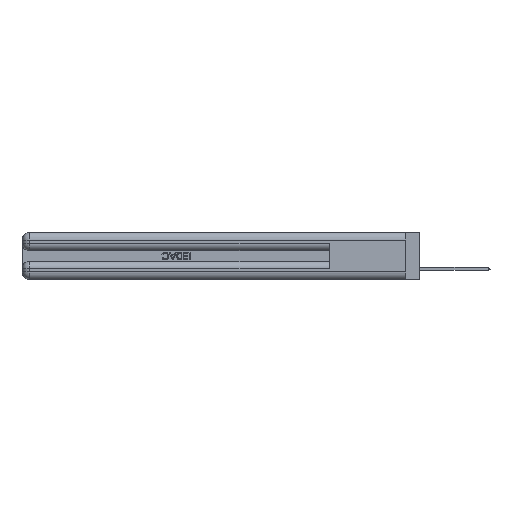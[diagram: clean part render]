
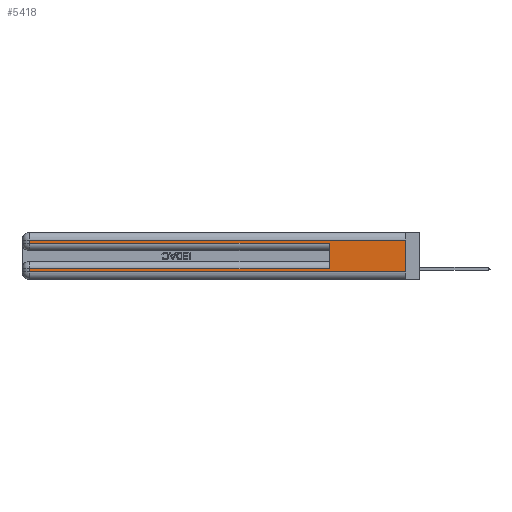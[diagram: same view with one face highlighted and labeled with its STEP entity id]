
A CAD part, left-side view. The second image highlights one B-rep face of the part: STEP entity #5418.
In plain terms, the highlighted planar face has unit normal (-1, 0, 0).
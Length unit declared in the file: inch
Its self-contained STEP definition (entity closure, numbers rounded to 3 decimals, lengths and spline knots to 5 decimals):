
#578 = CARTESIAN_POINT ( 'NONE',  ( 0., 0., 0.31 ) ) ;
#2004 = CARTESIAN_POINT ( 'NONE',  ( 0., 0., 0.06 ) ) ;
#3283 = ORIENTED_EDGE ( 'NONE', *, *, #33619, .F. ) ;
#3835 = CARTESIAN_POINT ( 'NONE',  ( 0., 2.94, 0.085 ) ) ;
#4847 = CARTESIAN_POINT ( 'NONE',  ( 0., 0.6, 0.145 ) ) ;
#4891 = FACE_OUTER_BOUND ( 'NONE', #30828, .T. ) ;
#5418 = ADVANCED_FACE ( 'NONE', ( #4891 ), #45806, .F. ) ;
#5597 = LINE ( 'NONE', #6065, #46303 ) ;
#5659 = ORIENTED_EDGE ( 'NONE', *, *, #11687, .T. ) ;
#6065 = CARTESIAN_POINT ( 'NONE',  ( 0., 0., 0.06 ) ) ;
#8136 = CARTESIAN_POINT ( 'NONE',  ( 0., 0.6, 0.285 ) ) ;
#8319 = DIRECTION ( 'NONE',  ( 0., -1., 0. ) ) ;
#9728 = DIRECTION ( 'NONE',  ( 0., -1., 0. ) ) ;
#9933 = ORIENTED_EDGE ( 'NONE', *, *, #39784, .T. ) ;
#10001 = EDGE_CURVE ( 'NONE', #17465, #18333, #43535, .T. ) ;
#10147 = DIRECTION ( 'NONE',  ( 0., 0., -1. ) ) ;
#11687 = EDGE_CURVE ( 'NONE', #16791, #30083, #5597, .T. ) ;
#12102 = EDGE_CURVE ( 'NONE', #19989, #16791, #15691, .T. ) ;
#12674 = ORIENTED_EDGE ( 'NONE', *, *, #14709, .T. ) ;
#13587 = CARTESIAN_POINT ( 'NONE',  ( 0., 0., 0.37 ) ) ;
#14413 = CARTESIAN_POINT ( 'NONE',  ( 0., 2.94, 0.31 ) ) ;
#14709 = EDGE_CURVE ( 'NONE', #17465, #19989, #40581, .T. ) ;
#15691 = LINE ( 'NONE', #34721, #22446 ) ;
#15802 = EDGE_CURVE ( 'NONE', #34759, #30915, #16139, .T. ) ;
#16139 = LINE ( 'NONE', #44559, #42785 ) ;
#16165 = DIRECTION ( 'NONE',  ( 0., 1., 0. ) ) ;
#16599 = ORIENTED_EDGE ( 'NONE', *, *, #10001, .F. ) ;
#16791 = VERTEX_POINT ( 'NONE', #44982 ) ;
#17465 = VERTEX_POINT ( 'NONE', #32274 ) ;
#18333 = VERTEX_POINT ( 'NONE', #8136 ) ;
#18549 = ORIENTED_EDGE ( 'NONE', *, *, #39634, .T. ) ;
#19989 = VERTEX_POINT ( 'NONE', #3835 ) ;
#21308 = VECTOR ( 'NONE', #35297, 39.37008 ) ;
#21739 = DIRECTION ( 'NONE',  ( 0., 1., 0. ) ) ;
#22446 = VECTOR ( 'NONE', #45543, 39.37008 ) ;
#22933 = DIRECTION ( 'NONE',  ( 0., 0., -1. ) ) ;
#26005 = CARTESIAN_POINT ( 'NONE',  ( 0., 0., 0.285 ) ) ;
#26171 = DIRECTION ( 'NONE',  ( 0., 0., 1. ) ) ;
#26595 = VECTOR ( 'NONE', #26171, 39.37008 ) ;
#27523 = DIRECTION ( 'NONE',  ( 1., 0., 0. ) ) ;
#28692 = LINE ( 'NONE', #13587, #21308 ) ;
#29706 = CARTESIAN_POINT ( 'NONE',  ( 0., 2.94, 0.285 ) ) ;
#30083 = VERTEX_POINT ( 'NONE', #2004 ) ;
#30324 = LINE ( 'NONE', #31939, #45590 ) ;
#30828 = EDGE_LOOP ( 'NONE', ( #3283, #9933, #41014, #18549, #16599, #12674, #33425, #5659 ) ) ;
#30915 = VERTEX_POINT ( 'NONE', #29706 ) ;
#31939 = CARTESIAN_POINT ( 'NONE',  ( 0., 0., 0.31 ) ) ;
#32274 = CARTESIAN_POINT ( 'NONE',  ( 0., 0.6, 0.085 ) ) ;
#33425 = ORIENTED_EDGE ( 'NONE', *, *, #12102, .T. ) ;
#33619 = EDGE_CURVE ( 'NONE', #46067, #30083, #28692, .T. ) ;
#33727 = LINE ( 'NONE', #26005, #44964 ) ;
#34721 = CARTESIAN_POINT ( 'NONE',  ( 0., 2.94, 0.37 ) ) ;
#34759 = VERTEX_POINT ( 'NONE', #14413 ) ;
#35297 = DIRECTION ( 'NONE',  ( 0., 0., -1. ) ) ;
#37685 = CARTESIAN_POINT ( 'NONE',  ( 0., 0., 0.085 ) ) ;
#38572 = CARTESIAN_POINT ( 'NONE',  ( 0., 0., 0.37 ) ) ;
#39634 = EDGE_CURVE ( 'NONE', #30915, #18333, #33727, .T. ) ;
#39784 = EDGE_CURVE ( 'NONE', #46067, #34759, #30324, .T. ) ;
#40581 = LINE ( 'NONE', #37685, #42331 ) ;
#41014 = ORIENTED_EDGE ( 'NONE', *, *, #15802, .T. ) ;
#42331 = VECTOR ( 'NONE', #16165, 39.37008 ) ;
#42785 = VECTOR ( 'NONE', #22933, 39.37008 ) ;
#43535 = LINE ( 'NONE', #4847, #26595 ) ;
#43589 = AXIS2_PLACEMENT_3D ( 'NONE', #38572, #27523, #10147 ) ;
#44559 = CARTESIAN_POINT ( 'NONE',  ( 0., 2.94, 0.37 ) ) ;
#44964 = VECTOR ( 'NONE', #8319, 39.37008 ) ;
#44982 = CARTESIAN_POINT ( 'NONE',  ( 0., 2.94, 0.06 ) ) ;
#45543 = DIRECTION ( 'NONE',  ( 0., 0., -1. ) ) ;
#45590 = VECTOR ( 'NONE', #21739, 39.37008 ) ;
#45806 = PLANE ( 'NONE',  #43589 ) ;
#46067 = VERTEX_POINT ( 'NONE', #578 ) ;
#46303 = VECTOR ( 'NONE', #9728, 39.37008 ) ;
